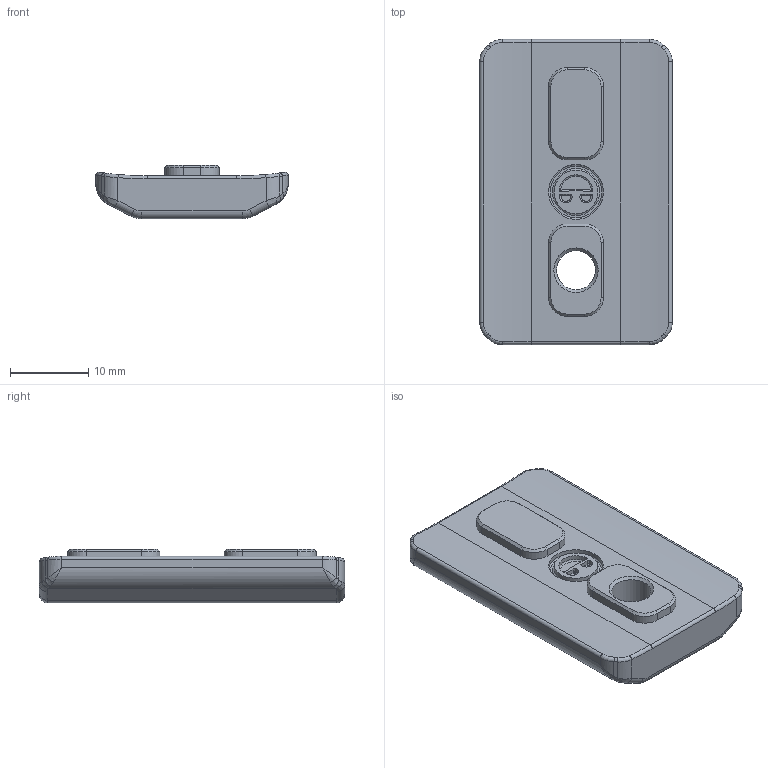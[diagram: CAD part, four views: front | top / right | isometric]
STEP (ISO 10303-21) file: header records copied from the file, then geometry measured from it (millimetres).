
FILE_DESCRIPTION(/* description */ (''),/* implementation_level */ '2;1');
FILE_NAME(/* name */ '1 Slot.step',/* time_stamp */ '2021-09-30T11:29:31-04:00',/* author */ (''),/* organization */ (''),/* preprocessor_version */ 'ST-DEVELOPER v18.1',/* originating_system */ 'Autodesk Translation Framework v10.10.0.1391',/* authorisation */ '');
FILE_SCHEMA (('AUTOMOTIVE_DESIGN { 1 0 10303 214 3 1 1 }'));
Length unit declared in the file: millimetre
Products named in the file (1): 1 Slot
Bounding box: 24.6 x 39 x 6.85 mm (x, y, z)
Volume: 4673.1 mm3; surface area: 2578.9 mm2
Topology: 1 solids, 1 shells, 144 faces, 327 edges, 189 vertices
Faces by surface type: cylinder 48, plane 36, bspline 30, torus 16, cone 10, sphere 4
Full cylindrical faces by diameter (mm): 5 x1, 5.6 x1, 7 x1, 9.3 x1
Entity records: 4562 total; most frequent: CARTESIAN_POINT 1357, DIRECTION 684, ORIENTED_EDGE 646, EDGE_CURVE 323, AXIS2_PLACEMENT_3D 282, VERTEX_POINT 189, EDGE_LOOP 154, FACE_OUTER_BOUND 144
